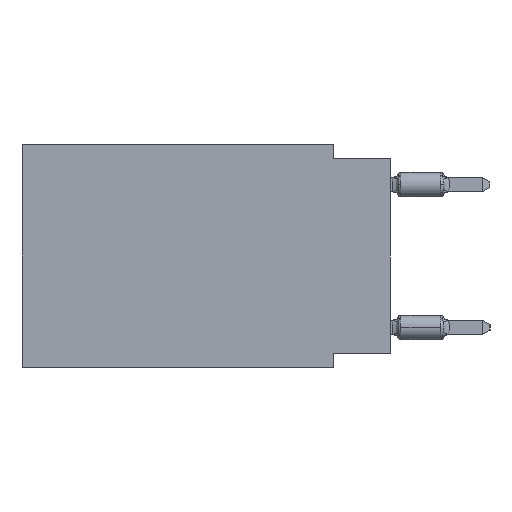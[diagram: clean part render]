
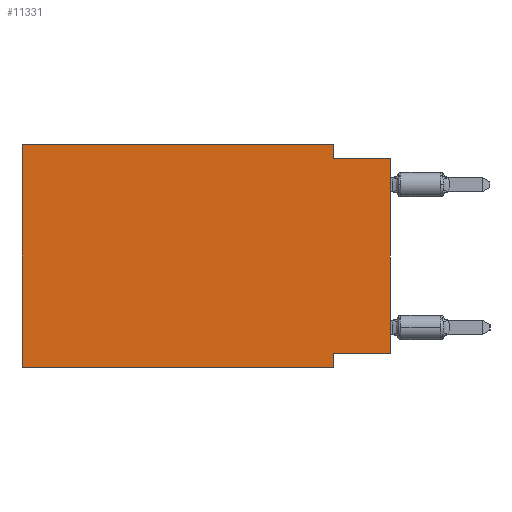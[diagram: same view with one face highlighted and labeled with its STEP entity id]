
A CAD part, left-side view. The second image highlights one B-rep face of the part: STEP entity #11331.
In plain terms, the highlighted planar face has unit normal (-1, 0, 0).
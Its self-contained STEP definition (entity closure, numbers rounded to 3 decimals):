
#21 = VERTEX_POINT ( 'NONE', #28231 ) ;
#1450 = VECTOR ( 'NONE', #22889, 1000. ) ;
#1943 = EDGE_CURVE ( 'NONE', #14478, #25975, #26443, .T. ) ;
#2926 = DIRECTION ( 'NONE',  ( 0., 0., 1. ) ) ;
#3640 = VECTOR ( 'NONE', #23236, 1000. ) ;
#3844 = DIRECTION ( 'NONE',  ( 1., 0., 0. ) ) ;
#3869 = ORIENTED_EDGE ( 'NONE', *, *, #24075, .T. ) ;
#4808 = LINE ( 'NONE', #5383, #20587 ) ;
#5188 = CARTESIAN_POINT ( 'NONE',  ( 0., 2.54, -9.271 ) ) ;
#5383 = CARTESIAN_POINT ( 'NONE',  ( 0., 0., 0. ) ) ;
#5385 = ORIENTED_EDGE ( 'NONE', *, *, #16837, .F. ) ;
#5538 = CARTESIAN_POINT ( 'NONE',  ( 0., 2.54, 0. ) ) ;
#5546 = EDGE_CURVE ( 'NONE', #22627, #9312, #4808, .T. ) ;
#5678 = LINE ( 'NONE', #5538, #5970 ) ;
#5970 = VECTOR ( 'NONE', #7875, 1000. ) ;
#6825 = CARTESIAN_POINT ( 'NONE',  ( 0., 2.54, -9.906 ) ) ;
#7535 = LINE ( 'NONE', #24901, #28567 ) ;
#7875 = DIRECTION ( 'NONE',  ( 0., 0., -1. ) ) ;
#8059 = FACE_OUTER_BOUND ( 'NONE', #13798, .T. ) ;
#8199 = CARTESIAN_POINT ( 'NONE',  ( 0., 16.383, -9.906 ) ) ;
#8784 = ORIENTED_EDGE ( 'NONE', *, *, #23218, .F. ) ;
#9220 = CARTESIAN_POINT ( 'NONE',  ( 0., 0., -0.635 ) ) ;
#9312 = VERTEX_POINT ( 'NONE', #9220 ) ;
#9945 = CARTESIAN_POINT ( 'NONE',  ( 0., 16.383, 0. ) ) ;
#10548 = CARTESIAN_POINT ( 'NONE',  ( 0., 2.54, -9.906 ) ) ;
#11268 = VERTEX_POINT ( 'NONE', #19832 ) ;
#11331 = ADVANCED_FACE ( 'NONE', ( #8059 ), #18758, .F. ) ;
#12244 = CARTESIAN_POINT ( 'NONE',  ( 0., 2.54, 0. ) ) ;
#12384 = DIRECTION ( 'NONE',  ( 0., -1., 0. ) ) ;
#12667 = DIRECTION ( 'NONE',  ( 0., 0., -1. ) ) ;
#13506 = EDGE_CURVE ( 'NONE', #21, #9312, #27567, .T. ) ;
#13798 = EDGE_LOOP ( 'NONE', ( #16964, #16250, #8784, #26677, #27378, #3869, #14304, #5385 ) ) ;
#14304 = ORIENTED_EDGE ( 'NONE', *, *, #1943, .F. ) ;
#14402 = LINE ( 'NONE', #23372, #26698 ) ;
#14478 = VERTEX_POINT ( 'NONE', #5188 ) ;
#15352 = VECTOR ( 'NONE', #21684, 1000. ) ;
#16011 = CARTESIAN_POINT ( 'NONE',  ( 0., 0., -0.635 ) ) ;
#16250 = ORIENTED_EDGE ( 'NONE', *, *, #13506, .F. ) ;
#16660 = CARTESIAN_POINT ( 'NONE',  ( 0., 0., -9.271 ) ) ;
#16837 = EDGE_CURVE ( 'NONE', #22627, #14478, #25063, .T. ) ;
#16964 = ORIENTED_EDGE ( 'NONE', *, *, #5546, .T. ) ;
#17900 = CARTESIAN_POINT ( 'NONE',  ( 0., 16.383, -9.906 ) ) ;
#18666 = DIRECTION ( 'NONE',  ( 0., 0., 1. ) ) ;
#18758 = PLANE ( 'NONE',  #24257 ) ;
#19656 = VERTEX_POINT ( 'NONE', #17900 ) ;
#19832 = CARTESIAN_POINT ( 'NONE',  ( 0., 16.383, 0. ) ) ;
#20587 = VECTOR ( 'NONE', #2926, 1000. ) ;
#21684 = DIRECTION ( 'NONE',  ( 0., 0., -1. ) ) ;
#22627 = VERTEX_POINT ( 'NONE', #25157 ) ;
#22889 = DIRECTION ( 'NONE',  ( 0., 1., 0. ) ) ;
#23218 = EDGE_CURVE ( 'NONE', #24102, #21, #5678, .T. ) ;
#23236 = DIRECTION ( 'NONE',  ( 0., -1., 0. ) ) ;
#23372 = CARTESIAN_POINT ( 'NONE',  ( 0., 16.383, 0. ) ) ;
#23650 = VECTOR ( 'NONE', #24842, 1000. ) ;
#24075 = EDGE_CURVE ( 'NONE', #19656, #25975, #27992, .T. ) ;
#24102 = VERTEX_POINT ( 'NONE', #12244 ) ;
#24257 = AXIS2_PLACEMENT_3D ( 'NONE', #9945, #3844, #12667 ) ;
#24842 = DIRECTION ( 'NONE',  ( 0., -1., 0. ) ) ;
#24901 = CARTESIAN_POINT ( 'NONE',  ( 0., 16.383, 0. ) ) ;
#25063 = LINE ( 'NONE', #16660, #1450 ) ;
#25157 = CARTESIAN_POINT ( 'NONE',  ( 0., 0., -9.271 ) ) ;
#25358 = EDGE_CURVE ( 'NONE', #11268, #24102, #14402, .T. ) ;
#25975 = VERTEX_POINT ( 'NONE', #6825 ) ;
#26443 = LINE ( 'NONE', #10548, #15352 ) ;
#26677 = ORIENTED_EDGE ( 'NONE', *, *, #25358, .F. ) ;
#26698 = VECTOR ( 'NONE', #12384, 1000. ) ;
#27378 = ORIENTED_EDGE ( 'NONE', *, *, #28179, .F. ) ;
#27567 = LINE ( 'NONE', #16011, #23650 ) ;
#27992 = LINE ( 'NONE', #8199, #3640 ) ;
#28179 = EDGE_CURVE ( 'NONE', #19656, #11268, #7535, .T. ) ;
#28231 = CARTESIAN_POINT ( 'NONE',  ( 0., 2.54, -0.635 ) ) ;
#28567 = VECTOR ( 'NONE', #18666, 1000. ) ;
